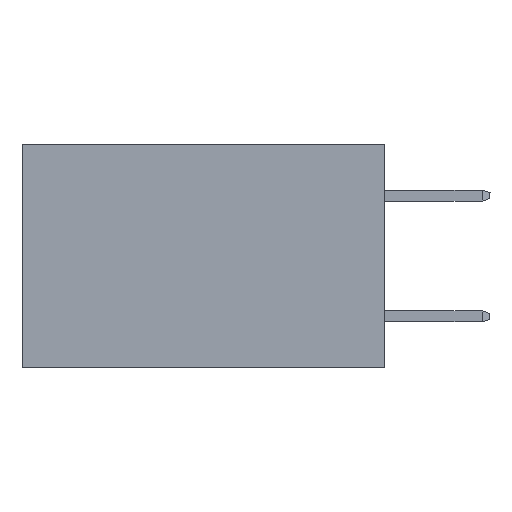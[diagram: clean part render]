
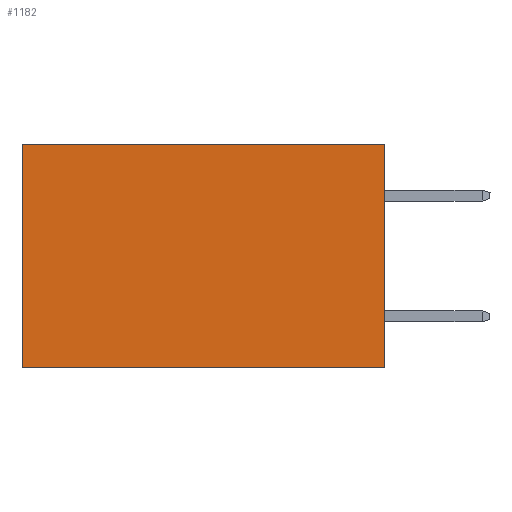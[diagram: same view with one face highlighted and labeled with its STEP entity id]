
A CAD part, left-side view. The second image highlights one B-rep face of the part: STEP entity #1182.
In plain terms, the highlighted planar face has unit normal (-1, 0, 0).
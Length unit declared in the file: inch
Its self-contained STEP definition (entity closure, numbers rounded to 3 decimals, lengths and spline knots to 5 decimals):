
#213 = ORIENTED_EDGE ( 'NONE', *, *, #14336, .F. ) ;
#411 = CARTESIAN_POINT ( 'NONE',  ( 0.298, 0., -0.37 ) ) ;
#1182 = ADVANCED_FACE ( 'NONE', ( #12170 ), #19908, .F. ) ;
#1524 = DIRECTION ( 'NONE',  ( 0., 0., -1. ) ) ;
#2405 = VERTEX_POINT ( 'NONE', #411 ) ;
#2582 = EDGE_CURVE ( 'NONE', #2405, #4737, #9701, .T. ) ;
#4286 = VECTOR ( 'NONE', #1524, 39.37008 ) ;
#4737 = VERTEX_POINT ( 'NONE', #11019 ) ;
#5238 = ORIENTED_EDGE ( 'NONE', *, *, #2582, .F. ) ;
#6239 = DIRECTION ( 'NONE',  ( 1., 0., 0. ) ) ;
#6538 = CARTESIAN_POINT ( 'NONE',  ( 0.298, 0., 0. ) ) ;
#7136 = VERTEX_POINT ( 'NONE', #20055 ) ;
#8051 = DIRECTION ( 'NONE',  ( 0., 0., -1. ) ) ;
#8855 = LINE ( 'NONE', #10022, #4286 ) ;
#9496 = EDGE_LOOP ( 'NONE', ( #18785, #5238, #213, #13361 ) ) ;
#9654 = CARTESIAN_POINT ( 'NONE',  ( 0.298, 0., 0. ) ) ;
#9701 = LINE ( 'NONE', #20283, #19526 ) ;
#10022 = CARTESIAN_POINT ( 'NONE',  ( 0.298, 0.6, 0. ) ) ;
#11019 = CARTESIAN_POINT ( 'NONE',  ( 0.298, 0.6, -0.37 ) ) ;
#11535 = LINE ( 'NONE', #6538, #12849 ) ;
#11814 = EDGE_CURVE ( 'NONE', #7136, #20251, #13737, .T. ) ;
#12170 = FACE_OUTER_BOUND ( 'NONE', #9496, .T. ) ;
#12849 = VECTOR ( 'NONE', #20056, 39.37008 ) ;
#13361 = ORIENTED_EDGE ( 'NONE', *, *, #11814, .T. ) ;
#13737 = LINE ( 'NONE', #20577, #14541 ) ;
#14336 = EDGE_CURVE ( 'NONE', #7136, #2405, #11535, .T. ) ;
#14395 = EDGE_CURVE ( 'NONE', #20251, #4737, #8855, .T. ) ;
#14541 = VECTOR ( 'NONE', #17436, 39.37008 ) ;
#15198 = DIRECTION ( 'NONE',  ( 0., 1., 0. ) ) ;
#17436 = DIRECTION ( 'NONE',  ( 0., 1., 0. ) ) ;
#17988 = AXIS2_PLACEMENT_3D ( 'NONE', #9654, #6239, #8051 ) ;
#18785 = ORIENTED_EDGE ( 'NONE', *, *, #14395, .T. ) ;
#19026 = CARTESIAN_POINT ( 'NONE',  ( 0.298, 0.6, 0. ) ) ;
#19526 = VECTOR ( 'NONE', #15198, 39.37008 ) ;
#19908 = PLANE ( 'NONE',  #17988 ) ;
#20055 = CARTESIAN_POINT ( 'NONE',  ( 0.298, 0., 0. ) ) ;
#20056 = DIRECTION ( 'NONE',  ( 0., 0., -1. ) ) ;
#20251 = VERTEX_POINT ( 'NONE', #19026 ) ;
#20283 = CARTESIAN_POINT ( 'NONE',  ( 0.298, 0., -0.37 ) ) ;
#20577 = CARTESIAN_POINT ( 'NONE',  ( 0.298, 0., 0. ) ) ;
